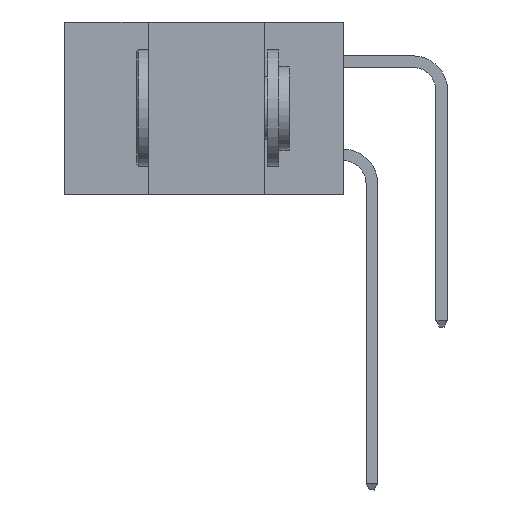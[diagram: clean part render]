
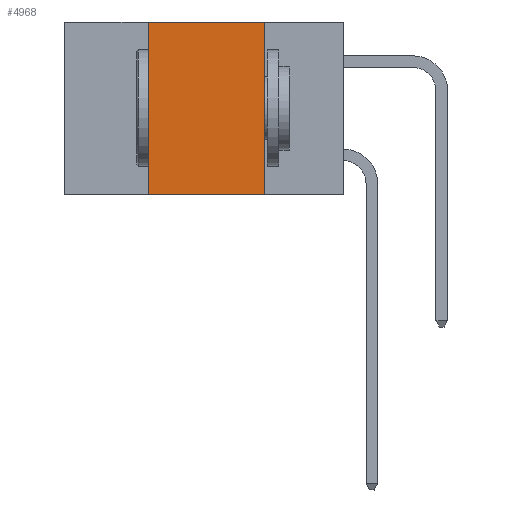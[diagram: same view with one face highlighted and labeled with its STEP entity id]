
A CAD part, left-side view. The second image highlights one B-rep face of the part: STEP entity #4968.
In plain terms, the highlighted planar face has unit normal (-1, 0, 0).
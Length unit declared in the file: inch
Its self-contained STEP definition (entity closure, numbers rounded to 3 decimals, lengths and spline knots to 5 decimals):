
#77 = DIRECTION ( 'NONE',  ( 0., -1., 0. ) ) ;
#327 = DIRECTION ( 'NONE',  ( 0., 0., 1. ) ) ;
#450 = PLANE ( 'NONE',  #6523 ) ;
#563 = VECTOR ( 'NONE', #2612, 39.37008 ) ;
#1062 = ORIENTED_EDGE ( 'NONE', *, *, #13839, .F. ) ;
#1546 = VERTEX_POINT ( 'NONE', #3013 ) ;
#2612 = DIRECTION ( 'NONE',  ( 0., 0., -1. ) ) ;
#3013 = CARTESIAN_POINT ( 'NONE',  ( 0., 0.17, -0.37 ) ) ;
#3029 = ORIENTED_EDGE ( 'NONE', *, *, #12430, .F. ) ;
#3966 = DIRECTION ( 'NONE',  ( 1., 0., 0. ) ) ;
#4111 = CARTESIAN_POINT ( 'NONE',  ( 0., 0.42, 0. ) ) ;
#4514 = VECTOR ( 'NONE', #327, 39.37008 ) ;
#4962 = EDGE_LOOP ( 'NONE', ( #6026, #1062, #3029, #10833 ) ) ;
#4968 = ADVANCED_FACE ( 'NONE', ( #14472 ), #450, .F. ) ;
#5072 = CARTESIAN_POINT ( 'NONE',  ( 0., 0.17, -0.37 ) ) ;
#5582 = LINE ( 'NONE', #13444, #13666 ) ;
#5927 = LINE ( 'NONE', #8238, #14086 ) ;
#6026 = ORIENTED_EDGE ( 'NONE', *, *, #10503, .F. ) ;
#6523 = AXIS2_PLACEMENT_3D ( 'NONE', #12225, #3966, #8677 ) ;
#6590 = VERTEX_POINT ( 'NONE', #4111 ) ;
#6632 = LINE ( 'NONE', #10938, #4514 ) ;
#7175 = LINE ( 'NONE', #5072, #563 ) ;
#8135 = CARTESIAN_POINT ( 'NONE',  ( 0., 0.17, 0. ) ) ;
#8238 = CARTESIAN_POINT ( 'NONE',  ( 0., 0.6, -0.37 ) ) ;
#8677 = DIRECTION ( 'NONE',  ( 0., 0., -1. ) ) ;
#10127 = DIRECTION ( 'NONE',  ( 0., -1., 0. ) ) ;
#10503 = EDGE_CURVE ( 'NONE', #11893, #1546, #7175, .T. ) ;
#10833 = ORIENTED_EDGE ( 'NONE', *, *, #10949, .T. ) ;
#10938 = CARTESIAN_POINT ( 'NONE',  ( 0., 0.42, -0.37 ) ) ;
#10949 = EDGE_CURVE ( 'NONE', #11351, #1546, #5927, .T. ) ;
#11351 = VERTEX_POINT ( 'NONE', #12913 ) ;
#11893 = VERTEX_POINT ( 'NONE', #8135 ) ;
#12225 = CARTESIAN_POINT ( 'NONE',  ( 0., 0.6, 0. ) ) ;
#12430 = EDGE_CURVE ( 'NONE', #11351, #6590, #6632, .T. ) ;
#12913 = CARTESIAN_POINT ( 'NONE',  ( 0., 0.42, -0.37 ) ) ;
#13444 = CARTESIAN_POINT ( 'NONE',  ( 0., 0.6, 0. ) ) ;
#13666 = VECTOR ( 'NONE', #10127, 39.37008 ) ;
#13839 = EDGE_CURVE ( 'NONE', #6590, #11893, #5582, .T. ) ;
#14086 = VECTOR ( 'NONE', #77, 39.37008 ) ;
#14472 = FACE_OUTER_BOUND ( 'NONE', #4962, .T. ) ;
